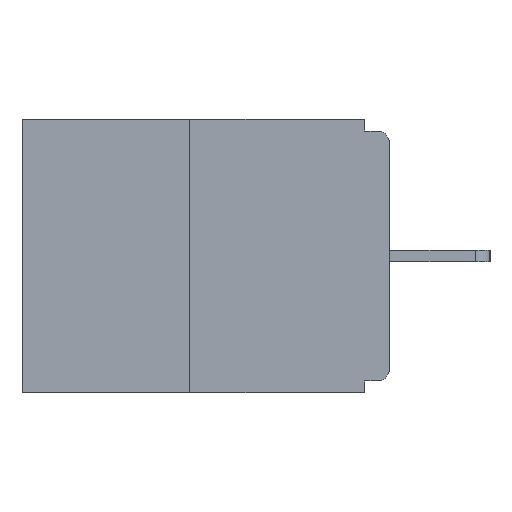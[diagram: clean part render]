
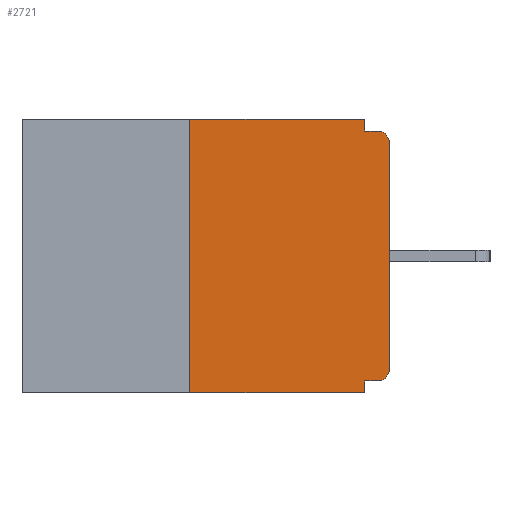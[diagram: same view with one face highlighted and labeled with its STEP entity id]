
A CAD part, left-side view. The second image highlights one B-rep face of the part: STEP entity #2721.
In plain terms, the highlighted planar face has unit normal (-1, 0, 0).
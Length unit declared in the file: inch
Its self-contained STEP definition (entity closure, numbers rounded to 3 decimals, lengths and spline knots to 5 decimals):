
#58 = CARTESIAN_POINT ( 'NONE',  ( 0., 0.25, 0. ) ) ;
#690 = FACE_OUTER_BOUND ( 'NONE', #4224, .T. ) ;
#816 = ORIENTED_EDGE ( 'NONE', *, *, #8427, .F. ) ;
#969 = CARTESIAN_POINT ( 'NONE',  ( 0., 0.25, 0. ) ) ;
#1050 = CARTESIAN_POINT ( 'NONE',  ( 0., 0.25, -0.343 ) ) ;
#1120 = LINE ( 'NONE', #8932, #12136 ) ;
#1205 = ORIENTED_EDGE ( 'NONE', *, *, #10849, .T. ) ;
#1206 = DIRECTION ( 'NONE',  ( 0., 0., -1. ) ) ;
#1600 = ORIENTED_EDGE ( 'NONE', *, *, #13236, .F. ) ;
#1977 = VERTEX_POINT ( 'NONE', #13280 ) ;
#2246 = VERTEX_POINT ( 'NONE', #5363 ) ;
#2721 = ADVANCED_FACE ( 'NONE', ( #690 ), #10365, .F. ) ;
#2896 = VERTEX_POINT ( 'NONE', #9022 ) ;
#3024 = LINE ( 'NONE', #3654, #12923 ) ;
#3191 = CARTESIAN_POINT ( 'NONE',  ( 0., 0.031, -0.015 ) ) ;
#3654 = CARTESIAN_POINT ( 'NONE',  ( 0., 0.031, -0.343 ) ) ;
#3690 = CARTESIAN_POINT ( 'NONE',  ( 0., 0., -0.313 ) ) ;
#4101 = ORIENTED_EDGE ( 'NONE', *, *, #10404, .F. ) ;
#4137 = CIRCLE ( 'NONE', #7393, 0.015 ) ;
#4224 = EDGE_LOOP ( 'NONE', ( #8919, #11375, #9208, #816, #4101, #1205, #9804, #12206, #1600, #5181 ) ) ;
#4326 = EDGE_CURVE ( 'NONE', #12828, #2896, #12330, .T. ) ;
#4801 = VECTOR ( 'NONE', #7769, 39.37008 ) ;
#4823 = AXIS2_PLACEMENT_3D ( 'NONE', #10063, #10909, #10857 ) ;
#4853 = VECTOR ( 'NONE', #12947, 39.37008 ) ;
#5181 = ORIENTED_EDGE ( 'NONE', *, *, #7173, .F. ) ;
#5242 = VERTEX_POINT ( 'NONE', #8507 ) ;
#5363 = CARTESIAN_POINT ( 'NONE',  ( 0., 0.015, -0.015 ) ) ;
#5423 = DIRECTION ( 'NONE',  ( -1., 0., 0. ) ) ;
#5738 = CARTESIAN_POINT ( 'NONE',  ( 0., 0.015, -0.313 ) ) ;
#6023 = VERTEX_POINT ( 'NONE', #3690 ) ;
#6192 = CARTESIAN_POINT ( 'NONE',  ( 0., 0., -0.015 ) ) ;
#6384 = LINE ( 'NONE', #6192, #8613 ) ;
#6777 = DIRECTION ( 'NONE',  ( 0., 0., -1. ) ) ;
#7017 = VECTOR ( 'NONE', #8344, 39.37008 ) ;
#7028 = VECTOR ( 'NONE', #8093, 39.37008 ) ;
#7038 = LINE ( 'NONE', #8417, #4853 ) ;
#7173 = EDGE_CURVE ( 'NONE', #2896, #7786, #1120, .T. ) ;
#7179 = DIRECTION ( 'NONE',  ( 0., -1., 0. ) ) ;
#7323 = LINE ( 'NONE', #7407, #7017 ) ;
#7393 = AXIS2_PLACEMENT_3D ( 'NONE', #11175, #5423, #12065 ) ;
#7407 = CARTESIAN_POINT ( 'NONE',  ( 0., 0., -0.328 ) ) ;
#7594 = LINE ( 'NONE', #7730, #4801 ) ;
#7730 = CARTESIAN_POINT ( 'NONE',  ( 0., 0., 0. ) ) ;
#7769 = DIRECTION ( 'NONE',  ( 0., 0., 1. ) ) ;
#7786 = VERTEX_POINT ( 'NONE', #3191 ) ;
#7902 = CARTESIAN_POINT ( 'NONE',  ( 0., 0., -0.03 ) ) ;
#8093 = DIRECTION ( 'NONE',  ( 0., 0., 1. ) ) ;
#8165 = VERTEX_POINT ( 'NONE', #1050 ) ;
#8344 = DIRECTION ( 'NONE',  ( 0., 1., 0. ) ) ;
#8417 = CARTESIAN_POINT ( 'NONE',  ( 0., 0.46, -0.343 ) ) ;
#8427 = EDGE_CURVE ( 'NONE', #13137, #5242, #3024, .T. ) ;
#8507 = CARTESIAN_POINT ( 'NONE',  ( 0., 0.031, -0.343 ) ) ;
#8613 = VECTOR ( 'NONE', #7179, 39.37008 ) ;
#8919 = ORIENTED_EDGE ( 'NONE', *, *, #4326, .F. ) ;
#8932 = CARTESIAN_POINT ( 'NONE',  ( 0., 0.031, 0. ) ) ;
#8988 = EDGE_CURVE ( 'NONE', #11251, #2246, #4137, .T. ) ;
#9022 = CARTESIAN_POINT ( 'NONE',  ( 0., 0.031, 0. ) ) ;
#9047 = AXIS2_PLACEMENT_3D ( 'NONE', #5738, #12297, #6777 ) ;
#9061 = EDGE_CURVE ( 'NONE', #8165, #5242, #7038, .T. ) ;
#9208 = ORIENTED_EDGE ( 'NONE', *, *, #9061, .T. ) ;
#9359 = CIRCLE ( 'NONE', #9047, 0.015 ) ;
#9431 = DIRECTION ( 'NONE',  ( 0., -1., 0. ) ) ;
#9680 = EDGE_CURVE ( 'NONE', #8165, #12828, #12224, .T. ) ;
#9804 = ORIENTED_EDGE ( 'NONE', *, *, #12785, .T. ) ;
#9871 = DIRECTION ( 'NONE',  ( 0., 0., -1. ) ) ;
#9940 = VECTOR ( 'NONE', #9431, 39.37008 ) ;
#10063 = CARTESIAN_POINT ( 'NONE',  ( 0., 0.46, 0. ) ) ;
#10365 = PLANE ( 'NONE',  #4823 ) ;
#10404 = EDGE_CURVE ( 'NONE', #1977, #13137, #7323, .T. ) ;
#10849 = EDGE_CURVE ( 'NONE', #1977, #6023, #9359, .T. ) ;
#10857 = DIRECTION ( 'NONE',  ( 0., 0., -1. ) ) ;
#10909 = DIRECTION ( 'NONE',  ( 1., 0., 0. ) ) ;
#11175 = CARTESIAN_POINT ( 'NONE',  ( 0., 0.015, -0.03 ) ) ;
#11251 = VERTEX_POINT ( 'NONE', #7902 ) ;
#11375 = ORIENTED_EDGE ( 'NONE', *, *, #9680, .F. ) ;
#11585 = CARTESIAN_POINT ( 'NONE',  ( 0., 0.031, -0.328 ) ) ;
#11669 = CARTESIAN_POINT ( 'NONE',  ( 0., 0.46, 0. ) ) ;
#12065 = DIRECTION ( 'NONE',  ( 0., 0., -1. ) ) ;
#12136 = VECTOR ( 'NONE', #9871, 39.37008 ) ;
#12206 = ORIENTED_EDGE ( 'NONE', *, *, #8988, .T. ) ;
#12224 = LINE ( 'NONE', #58, #7028 ) ;
#12297 = DIRECTION ( 'NONE',  ( -1., 0., 0. ) ) ;
#12330 = LINE ( 'NONE', #11669, #9940 ) ;
#12785 = EDGE_CURVE ( 'NONE', #6023, #11251, #7594, .T. ) ;
#12828 = VERTEX_POINT ( 'NONE', #969 ) ;
#12923 = VECTOR ( 'NONE', #1206, 39.37008 ) ;
#12947 = DIRECTION ( 'NONE',  ( 0., -1., 0. ) ) ;
#13137 = VERTEX_POINT ( 'NONE', #11585 ) ;
#13236 = EDGE_CURVE ( 'NONE', #7786, #2246, #6384, .T. ) ;
#13280 = CARTESIAN_POINT ( 'NONE',  ( 0., 0.015, -0.328 ) ) ;
